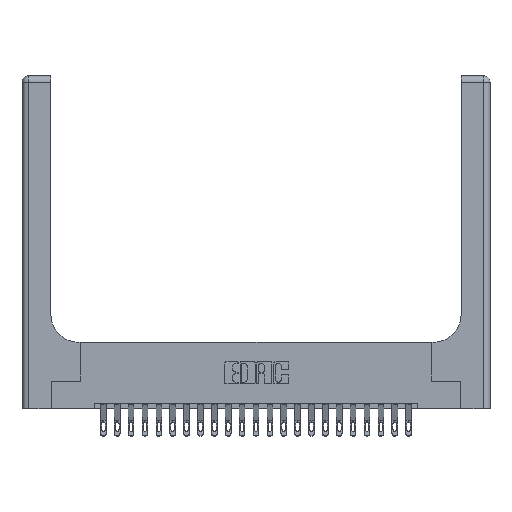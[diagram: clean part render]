
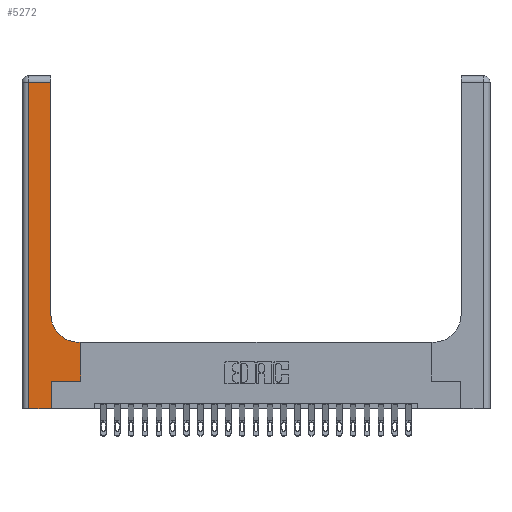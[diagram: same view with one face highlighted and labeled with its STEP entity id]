
A CAD part, top view. The second image highlights one B-rep face of the part: STEP entity #5272.
In plain terms, the highlighted planar face has unit normal (0, 0, 1).
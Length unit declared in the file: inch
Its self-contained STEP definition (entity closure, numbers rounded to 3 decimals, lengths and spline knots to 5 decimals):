
#521 = VECTOR ( 'NONE', #15992, 39.37008 ) ;
#796 = EDGE_CURVE ( 'NONE', #9159, #17054, #15910, .T. ) ;
#1012 = VERTEX_POINT ( 'NONE', #16449 ) ;
#1362 = ORIENTED_EDGE ( 'NONE', *, *, #23038, .T. ) ;
#1602 = DIRECTION ( 'NONE',  ( 0., 1., 0. ) ) ;
#2129 = CARTESIAN_POINT ( 'NONE',  ( 0.06, 0., 0.37 ) ) ;
#2725 = DIRECTION ( 'NONE',  ( 0., 0., -1. ) ) ;
#2789 = VERTEX_POINT ( 'NONE', #17352 ) ;
#3546 = PLANE ( 'NONE',  #15512 ) ;
#3852 = VECTOR ( 'NONE', #6858, 39.37008 ) ;
#4581 = CIRCLE ( 'NONE', #17884, 0.25 ) ;
#5065 = VERTEX_POINT ( 'NONE', #6764 ) ;
#5219 = CARTESIAN_POINT ( 'NONE',  ( 0.06, 2.94, 0.37 ) ) ;
#5231 = VERTEX_POINT ( 'NONE', #5219 ) ;
#5272 = ADVANCED_FACE ( 'NONE', ( #12608 ), #3546, .F. ) ;
#5584 = VERTEX_POINT ( 'NONE', #16127 ) ;
#6093 = EDGE_CURVE ( 'NONE', #5584, #15336, #8727, .T. ) ;
#6215 = EDGE_CURVE ( 'NONE', #2789, #5065, #4581, .T. ) ;
#6639 = LINE ( 'NONE', #8310, #19237 ) ;
#6764 = CARTESIAN_POINT ( 'NONE',  ( 0.26, 0.85, 0.37 ) ) ;
#6828 = DIRECTION ( 'NONE',  ( 1., 0., 0. ) ) ;
#6858 = DIRECTION ( 'NONE',  ( 1., 0., 0. ) ) ;
#6898 = EDGE_CURVE ( 'NONE', #17054, #5584, #7326, .T. ) ;
#7197 = LINE ( 'NONE', #12687, #9945 ) ;
#7326 = LINE ( 'NONE', #17807, #10244 ) ;
#7849 = ORIENTED_EDGE ( 'NONE', *, *, #19721, .T. ) ;
#7933 = EDGE_LOOP ( 'NONE', ( #17012, #7849, #20784, #12866, #12360, #23492, #1362, #17959, #9745 ) ) ;
#8067 = DIRECTION ( 'NONE',  ( -1., 0., 0. ) ) ;
#8074 = DIRECTION ( 'NONE',  ( 1., 0., 0. ) ) ;
#8310 = CARTESIAN_POINT ( 'NONE',  ( 0., 2.94, 0.37 ) ) ;
#8599 = CARTESIAN_POINT ( 'NONE',  ( 0.26, 2.94, 0.37 ) ) ;
#8727 = LINE ( 'NONE', #16100, #19016 ) ;
#9159 = VERTEX_POINT ( 'NONE', #2129 ) ;
#9369 = LINE ( 'NONE', #19863, #15447 ) ;
#9745 = ORIENTED_EDGE ( 'NONE', *, *, #6215, .T. ) ;
#9945 = VECTOR ( 'NONE', #1602, 39.37008 ) ;
#10115 = LINE ( 'NONE', #12029, #14678 ) ;
#10244 = VECTOR ( 'NONE', #12584, 39.37008 ) ;
#10809 = DIRECTION ( 'NONE',  ( 0., 0., -1. ) ) ;
#11908 = DIRECTION ( 'NONE',  ( -1., 0., 0. ) ) ;
#12029 = CARTESIAN_POINT ( 'NONE',  ( 0.26, 0.6, 0.37 ) ) ;
#12360 = ORIENTED_EDGE ( 'NONE', *, *, #6898, .T. ) ;
#12584 = DIRECTION ( 'NONE',  ( 0., 1., 0. ) ) ;
#12608 = FACE_OUTER_BOUND ( 'NONE', #7933, .T. ) ;
#12687 = CARTESIAN_POINT ( 'NONE',  ( 0.528, 0.25, 0.37 ) ) ;
#12730 = CARTESIAN_POINT ( 'NONE',  ( 0.265, 0., 0.37 ) ) ;
#12842 = CARTESIAN_POINT ( 'NONE',  ( 0., 3., 0.37 ) ) ;
#12866 = ORIENTED_EDGE ( 'NONE', *, *, #796, .T. ) ;
#14512 = EDGE_CURVE ( 'NONE', #5231, #9159, #19560, .T. ) ;
#14678 = VECTOR ( 'NONE', #11908, 39.37008 ) ;
#15336 = VERTEX_POINT ( 'NONE', #15681 ) ;
#15342 = CARTESIAN_POINT ( 'NONE',  ( 0.51, 0.85, 0.37 ) ) ;
#15447 = VECTOR ( 'NONE', #18064, 39.37008 ) ;
#15512 = AXIS2_PLACEMENT_3D ( 'NONE', #12842, #10809, #20078 ) ;
#15681 = CARTESIAN_POINT ( 'NONE',  ( 0.528, 0.25, 0.37 ) ) ;
#15910 = LINE ( 'NONE', #23165, #3852 ) ;
#15992 = DIRECTION ( 'NONE',  ( 0., -1., 0. ) ) ;
#16100 = CARTESIAN_POINT ( 'NONE',  ( 0.265, 0.25, 0.37 ) ) ;
#16127 = CARTESIAN_POINT ( 'NONE',  ( 0.265, 0.25, 0.37 ) ) ;
#16449 = CARTESIAN_POINT ( 'NONE',  ( 0.528, 0.6, 0.37 ) ) ;
#16707 = EDGE_CURVE ( 'NONE', #1012, #2789, #10115, .T. ) ;
#17012 = ORIENTED_EDGE ( 'NONE', *, *, #17055, .T. ) ;
#17054 = VERTEX_POINT ( 'NONE', #12730 ) ;
#17055 = EDGE_CURVE ( 'NONE', #5065, #17532, #9369, .T. ) ;
#17352 = CARTESIAN_POINT ( 'NONE',  ( 0.51, 0.6, 0.37 ) ) ;
#17532 = VERTEX_POINT ( 'NONE', #8599 ) ;
#17807 = CARTESIAN_POINT ( 'NONE',  ( 0.265, 0., 0.37 ) ) ;
#17884 = AXIS2_PLACEMENT_3D ( 'NONE', #15342, #2725, #8074 ) ;
#17959 = ORIENTED_EDGE ( 'NONE', *, *, #16707, .T. ) ;
#18064 = DIRECTION ( 'NONE',  ( 0., 1., 0. ) ) ;
#19016 = VECTOR ( 'NONE', #6828, 39.37008 ) ;
#19237 = VECTOR ( 'NONE', #8067, 39.37008 ) ;
#19560 = LINE ( 'NONE', #23361, #521 ) ;
#19721 = EDGE_CURVE ( 'NONE', #17532, #5231, #6639, .T. ) ;
#19863 = CARTESIAN_POINT ( 'NONE',  ( 0.26, 3., 0.37 ) ) ;
#20078 = DIRECTION ( 'NONE',  ( -1., 0., 0. ) ) ;
#20784 = ORIENTED_EDGE ( 'NONE', *, *, #14512, .T. ) ;
#23038 = EDGE_CURVE ( 'NONE', #15336, #1012, #7197, .T. ) ;
#23165 = CARTESIAN_POINT ( 'NONE',  ( 0., 0., 0.37 ) ) ;
#23361 = CARTESIAN_POINT ( 'NONE',  ( 0.06, 3., 0.37 ) ) ;
#23492 = ORIENTED_EDGE ( 'NONE', *, *, #6093, .T. ) ;
